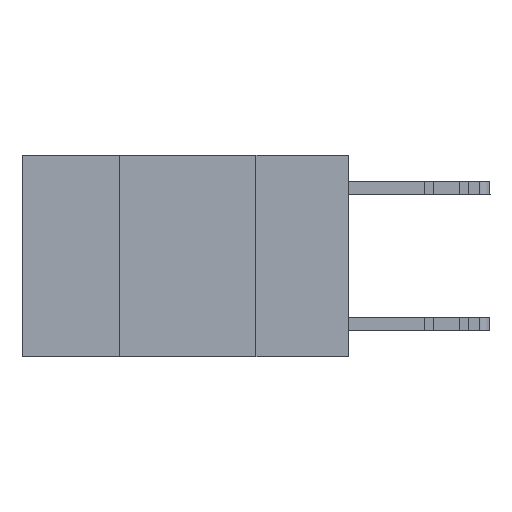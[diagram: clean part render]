
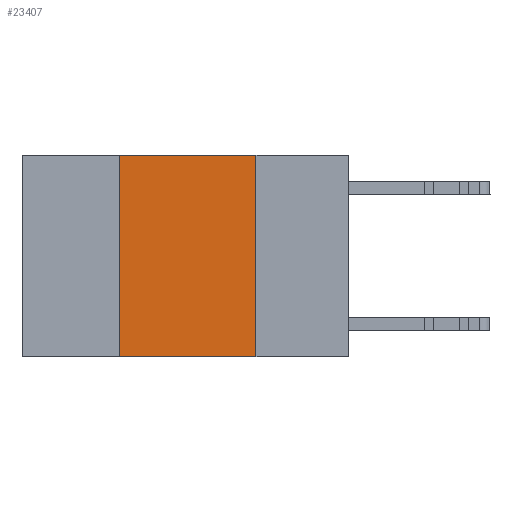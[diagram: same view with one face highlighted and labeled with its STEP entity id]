
A CAD part, left-side view. The second image highlights one B-rep face of the part: STEP entity #23407.
In plain terms, the highlighted planar face has unit normal (-1, 0, 0).
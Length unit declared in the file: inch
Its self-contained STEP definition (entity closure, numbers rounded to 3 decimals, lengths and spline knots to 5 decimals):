
#184 = EDGE_CURVE ( 'NONE', #22213, #7972, #22854, .T. ) ;
#925 = DIRECTION ( 'NONE',  ( 0., 0., 1. ) ) ;
#1092 = DIRECTION ( 'NONE',  ( 0., -1., 0. ) ) ;
#2546 = CARTESIAN_POINT ( 'NONE',  ( 0., 0.17, 0. ) ) ;
#4032 = CARTESIAN_POINT ( 'NONE',  ( 0., 0.42, 0. ) ) ;
#4299 = CARTESIAN_POINT ( 'NONE',  ( 0., 0.17, -0.37 ) ) ;
#5077 = LINE ( 'NONE', #11986, #16015 ) ;
#5827 = VECTOR ( 'NONE', #12107, 39.37008 ) ;
#5848 = FACE_OUTER_BOUND ( 'NONE', #25167, .T. ) ;
#5910 = LINE ( 'NONE', #12561, #5827 ) ;
#6200 = AXIS2_PLACEMENT_3D ( 'NONE', #9857, #25301, #11991 ) ;
#6756 = VERTEX_POINT ( 'NONE', #4299 ) ;
#7634 = ORIENTED_EDGE ( 'NONE', *, *, #11899, .F. ) ;
#7909 = CARTESIAN_POINT ( 'NONE',  ( 0., 0.42, 0. ) ) ;
#7972 = VERTEX_POINT ( 'NONE', #4032 ) ;
#9013 = VECTOR ( 'NONE', #17748, 39.37008 ) ;
#9215 = LINE ( 'NONE', #15498, #9013 ) ;
#9857 = CARTESIAN_POINT ( 'NONE',  ( 0., 0.6, 0. ) ) ;
#10433 = ORIENTED_EDGE ( 'NONE', *, *, #184, .F. ) ;
#11899 = EDGE_CURVE ( 'NONE', #28016, #6756, #5910, .T. ) ;
#11986 = CARTESIAN_POINT ( 'NONE',  ( 0., 0.6, 0. ) ) ;
#11991 = DIRECTION ( 'NONE',  ( 0., 0., -1. ) ) ;
#12107 = DIRECTION ( 'NONE',  ( 0., 0., -1. ) ) ;
#12561 = CARTESIAN_POINT ( 'NONE',  ( 0., 0.17, 0. ) ) ;
#15498 = CARTESIAN_POINT ( 'NONE',  ( 0., 0.6, -0.37 ) ) ;
#16015 = VECTOR ( 'NONE', #1092, 39.37008 ) ;
#17748 = DIRECTION ( 'NONE',  ( 0., -1., 0. ) ) ;
#19366 = CARTESIAN_POINT ( 'NONE',  ( 0., 0.42, -0.37 ) ) ;
#20948 = EDGE_CURVE ( 'NONE', #22213, #6756, #9215, .T. ) ;
#22213 = VERTEX_POINT ( 'NONE', #19366 ) ;
#22748 = VECTOR ( 'NONE', #925, 39.37008 ) ;
#22854 = LINE ( 'NONE', #7909, #22748 ) ;
#23407 = ADVANCED_FACE ( 'NONE', ( #5848 ), #25199, .F. ) ;
#25167 = EDGE_LOOP ( 'NONE', ( #7634, #28505, #10433, #26051 ) ) ;
#25199 = PLANE ( 'NONE',  #6200 ) ;
#25301 = DIRECTION ( 'NONE',  ( 1., 0., 0. ) ) ;
#26051 = ORIENTED_EDGE ( 'NONE', *, *, #20948, .T. ) ;
#26229 = EDGE_CURVE ( 'NONE', #7972, #28016, #5077, .T. ) ;
#28016 = VERTEX_POINT ( 'NONE', #2546 ) ;
#28505 = ORIENTED_EDGE ( 'NONE', *, *, #26229, .F. ) ;
